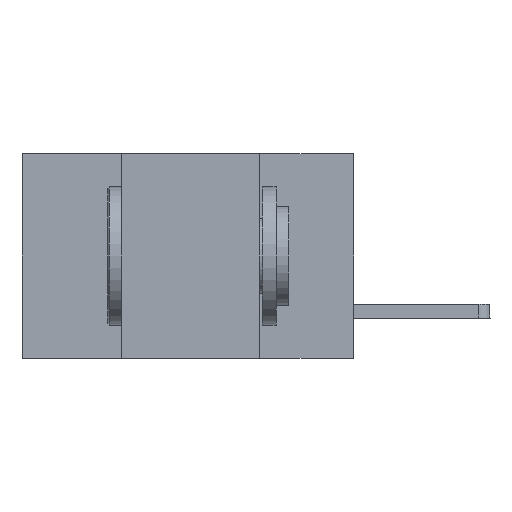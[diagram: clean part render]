
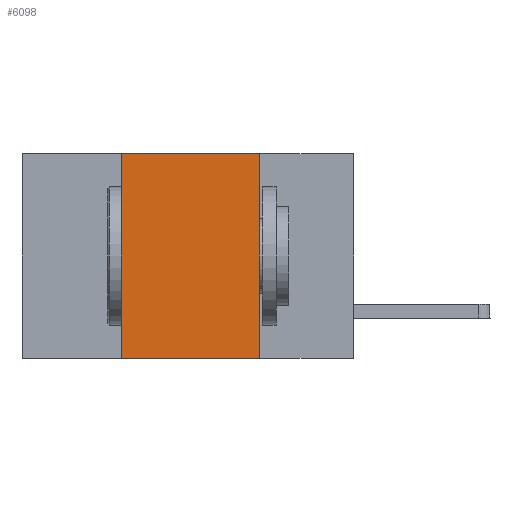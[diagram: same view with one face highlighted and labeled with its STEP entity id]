
A CAD part, left-side view. The second image highlights one B-rep face of the part: STEP entity #6098.
In plain terms, the highlighted planar face has unit normal (-1, 0, 0).
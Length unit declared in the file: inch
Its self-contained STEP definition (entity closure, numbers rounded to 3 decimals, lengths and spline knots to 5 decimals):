
#74 = CARTESIAN_POINT ( 'NONE',  ( 0., 0.6, -0.37 ) ) ;
#807 = ORIENTED_EDGE ( 'NONE', *, *, #3971, .F. ) ;
#1096 = CARTESIAN_POINT ( 'NONE',  ( 0., 0.6, 0. ) ) ;
#1483 = EDGE_LOOP ( 'NONE', ( #807, #4514, #6977, #11429 ) ) ;
#1547 = VECTOR ( 'NONE', #8477, 39.37008 ) ;
#1944 = CARTESIAN_POINT ( 'NONE',  ( 0., 0.42, -0.37 ) ) ;
#2718 = DIRECTION ( 'NONE',  ( 0., 0., -1. ) ) ;
#3307 = EDGE_CURVE ( 'NONE', #12250, #11411, #10179, .T. ) ;
#3313 = VERTEX_POINT ( 'NONE', #11099 ) ;
#3705 = DIRECTION ( 'NONE',  ( 0., 0., -1. ) ) ;
#3971 = EDGE_CURVE ( 'NONE', #3313, #11411, #6909, .T. ) ;
#4039 = VECTOR ( 'NONE', #8205, 39.37008 ) ;
#4507 = CARTESIAN_POINT ( 'NONE',  ( 0., 0.6, 0. ) ) ;
#4514 = ORIENTED_EDGE ( 'NONE', *, *, #9220, .F. ) ;
#5382 = LINE ( 'NONE', #1096, #10751 ) ;
#5592 = CARTESIAN_POINT ( 'NONE',  ( 0., 0.17, -0.37 ) ) ;
#5713 = LINE ( 'NONE', #12552, #1547 ) ;
#6098 = ADVANCED_FACE ( 'NONE', ( #12553 ), #6513, .F. ) ;
#6513 = PLANE ( 'NONE',  #9217 ) ;
#6909 = LINE ( 'NONE', #12026, #8013 ) ;
#6977 = ORIENTED_EDGE ( 'NONE', *, *, #8367, .F. ) ;
#7750 = DIRECTION ( 'NONE',  ( 1., 0., 0. ) ) ;
#8013 = VECTOR ( 'NONE', #2718, 39.37008 ) ;
#8205 = DIRECTION ( 'NONE',  ( 0., -1., 0. ) ) ;
#8367 = EDGE_CURVE ( 'NONE', #12250, #11021, #5713, .T. ) ;
#8402 = CARTESIAN_POINT ( 'NONE',  ( 0., 0.42, 0. ) ) ;
#8415 = DIRECTION ( 'NONE',  ( 0., -1., 0. ) ) ;
#8477 = DIRECTION ( 'NONE',  ( 0., 0., 1. ) ) ;
#9217 = AXIS2_PLACEMENT_3D ( 'NONE', #4507, #7750, #3705 ) ;
#9220 = EDGE_CURVE ( 'NONE', #11021, #3313, #5382, .T. ) ;
#10179 = LINE ( 'NONE', #74, #4039 ) ;
#10751 = VECTOR ( 'NONE', #8415, 39.37008 ) ;
#11021 = VERTEX_POINT ( 'NONE', #8402 ) ;
#11099 = CARTESIAN_POINT ( 'NONE',  ( 0., 0.17, 0. ) ) ;
#11411 = VERTEX_POINT ( 'NONE', #5592 ) ;
#11429 = ORIENTED_EDGE ( 'NONE', *, *, #3307, .T. ) ;
#12026 = CARTESIAN_POINT ( 'NONE',  ( 0., 0.17, 0. ) ) ;
#12250 = VERTEX_POINT ( 'NONE', #1944 ) ;
#12552 = CARTESIAN_POINT ( 'NONE',  ( 0., 0.42, 0. ) ) ;
#12553 = FACE_OUTER_BOUND ( 'NONE', #1483, .T. ) ;
